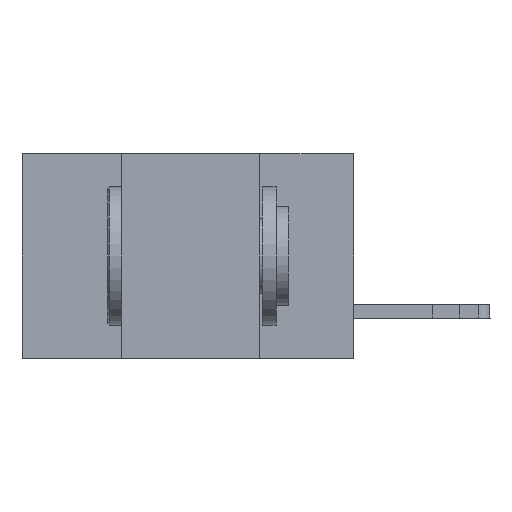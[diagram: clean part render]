
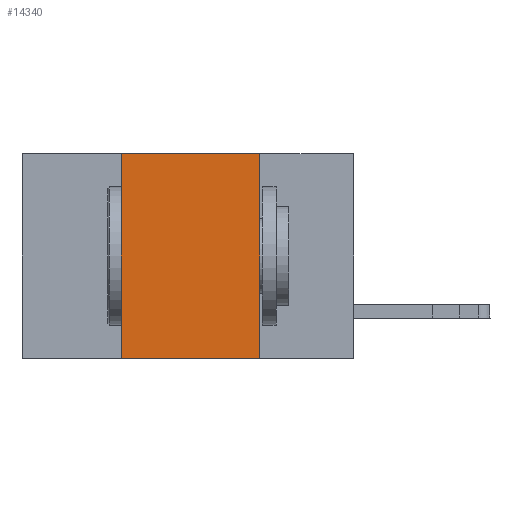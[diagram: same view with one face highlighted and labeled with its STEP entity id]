
A CAD part, left-side view. The second image highlights one B-rep face of the part: STEP entity #14340.
In plain terms, the highlighted planar face has unit normal (-1, 0, 0).
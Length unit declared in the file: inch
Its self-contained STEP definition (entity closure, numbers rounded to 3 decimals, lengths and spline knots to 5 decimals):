
#706 = EDGE_LOOP ( 'NONE', ( #11595, #20063, #21368, #10266 ) ) ;
#2064 = LINE ( 'NONE', #33262, #29391 ) ;
#3305 = LINE ( 'NONE', #25219, #23557 ) ;
#4325 = VERTEX_POINT ( 'NONE', #20397 ) ;
#4924 = DIRECTION ( 'NONE',  ( 0., 0., 1. ) ) ;
#5068 = CARTESIAN_POINT ( 'NONE',  ( 0., 0.6, -0.37 ) ) ;
#6728 = DIRECTION ( 'NONE',  ( 0., 0., -1. ) ) ;
#6905 = CARTESIAN_POINT ( 'NONE',  ( 0., 0.6, 0. ) ) ;
#7620 = DIRECTION ( 'NONE',  ( 0., -1., 0. ) ) ;
#7848 = VECTOR ( 'NONE', #4924, 39.37008 ) ;
#8418 = EDGE_CURVE ( 'NONE', #29967, #4325, #2064, .T. ) ;
#8454 = AXIS2_PLACEMENT_3D ( 'NONE', #6905, #9591, #28084 ) ;
#8699 = LINE ( 'NONE', #17849, #7848 ) ;
#9544 = LINE ( 'NONE', #5068, #29800 ) ;
#9591 = DIRECTION ( 'NONE',  ( 1., 0., 0. ) ) ;
#10266 = ORIENTED_EDGE ( 'NONE', *, *, #18786, .T. ) ;
#11595 = ORIENTED_EDGE ( 'NONE', *, *, #27489, .F. ) ;
#14340 = ADVANCED_FACE ( 'NONE', ( #33006 ), #22706, .F. ) ;
#15099 = VERTEX_POINT ( 'NONE', #17814 ) ;
#17814 = CARTESIAN_POINT ( 'NONE',  ( 0., 0.17, -0.37 ) ) ;
#17849 = CARTESIAN_POINT ( 'NONE',  ( 0., 0.42, 0. ) ) ;
#18786 = EDGE_CURVE ( 'NONE', #33790, #15099, #9544, .T. ) ;
#19234 = EDGE_CURVE ( 'NONE', #33790, #29967, #8699, .T. ) ;
#20063 = ORIENTED_EDGE ( 'NONE', *, *, #8418, .F. ) ;
#20397 = CARTESIAN_POINT ( 'NONE',  ( 0., 0.17, 0. ) ) ;
#21368 = ORIENTED_EDGE ( 'NONE', *, *, #19234, .F. ) ;
#22706 = PLANE ( 'NONE',  #8454 ) ;
#23557 = VECTOR ( 'NONE', #6728, 39.37008 ) ;
#25219 = CARTESIAN_POINT ( 'NONE',  ( 0., 0.17, 0. ) ) ;
#27489 = EDGE_CURVE ( 'NONE', #4325, #15099, #3305, .T. ) ;
#28084 = DIRECTION ( 'NONE',  ( 0., 0., -1. ) ) ;
#29391 = VECTOR ( 'NONE', #30772, 39.37008 ) ;
#29787 = CARTESIAN_POINT ( 'NONE',  ( 0., 0.42, 0. ) ) ;
#29800 = VECTOR ( 'NONE', #7620, 39.37008 ) ;
#29967 = VERTEX_POINT ( 'NONE', #29787 ) ;
#30772 = DIRECTION ( 'NONE',  ( 0., -1., 0. ) ) ;
#33006 = FACE_OUTER_BOUND ( 'NONE', #706, .T. ) ;
#33262 = CARTESIAN_POINT ( 'NONE',  ( 0., 0.6, 0. ) ) ;
#33508 = CARTESIAN_POINT ( 'NONE',  ( 0., 0.42, -0.37 ) ) ;
#33790 = VERTEX_POINT ( 'NONE', #33508 ) ;
